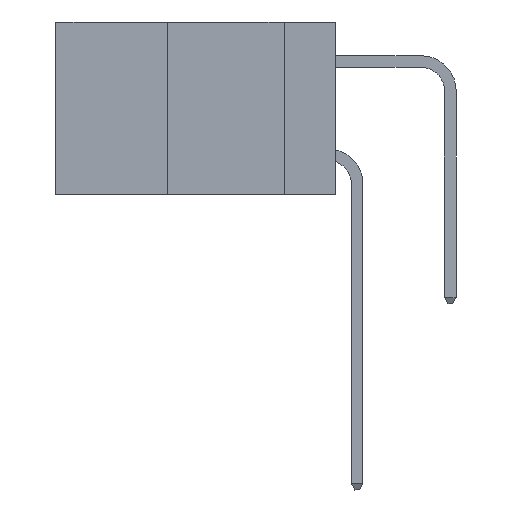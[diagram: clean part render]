
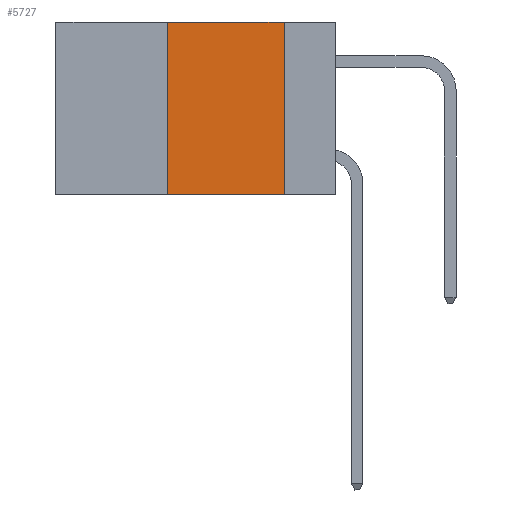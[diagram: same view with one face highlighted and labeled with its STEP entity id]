
A CAD part, left-side view. The second image highlights one B-rep face of the part: STEP entity #5727.
In plain terms, the highlighted planar face has unit normal (-1, 0, 0).
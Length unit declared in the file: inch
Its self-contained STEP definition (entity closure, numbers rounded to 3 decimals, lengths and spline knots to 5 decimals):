
#483 = VERTEX_POINT ( 'NONE', #3583 ) ;
#616 = DIRECTION ( 'NONE',  ( 1., 0., 0. ) ) ;
#626 = LINE ( 'NONE', #9694, #8537 ) ;
#1663 = ORIENTED_EDGE ( 'NONE', *, *, #20720, .F. ) ;
#2254 = LINE ( 'NONE', #4422, #19535 ) ;
#2584 = ORIENTED_EDGE ( 'NONE', *, *, #5345, .F. ) ;
#3583 = CARTESIAN_POINT ( 'NONE',  ( 0., 0.36, -0.37 ) ) ;
#4422 = CARTESIAN_POINT ( 'NONE',  ( 0., 0.11, 0. ) ) ;
#5345 = EDGE_CURVE ( 'NONE', #483, #9402, #626, .T. ) ;
#5434 = EDGE_CURVE ( 'NONE', #483, #13383, #18441, .T. ) ;
#5591 = FACE_OUTER_BOUND ( 'NONE', #19784, .T. ) ;
#5607 = CARTESIAN_POINT ( 'NONE',  ( 0., 0.6, 0. ) ) ;
#5727 = ADVANCED_FACE ( 'NONE', ( #5591 ), #17321, .F. ) ;
#5816 = ORIENTED_EDGE ( 'NONE', *, *, #11416, .F. ) ;
#7896 = CARTESIAN_POINT ( 'NONE',  ( 0., 0.11, 0. ) ) ;
#8312 = CARTESIAN_POINT ( 'NONE',  ( 0., 0.11, -0.37 ) ) ;
#8537 = VECTOR ( 'NONE', #13044, 39.37008 ) ;
#9402 = VERTEX_POINT ( 'NONE', #16211 ) ;
#9694 = CARTESIAN_POINT ( 'NONE',  ( 0., 0.36, 0. ) ) ;
#11203 = ORIENTED_EDGE ( 'NONE', *, *, #5434, .T. ) ;
#11416 = EDGE_CURVE ( 'NONE', #11446, #13383, #2254, .T. ) ;
#11446 = VERTEX_POINT ( 'NONE', #7896 ) ;
#12373 = DIRECTION ( 'NONE',  ( 0., 0., -1. ) ) ;
#13044 = DIRECTION ( 'NONE',  ( 0., 0., 1. ) ) ;
#13383 = VERTEX_POINT ( 'NONE', #8312 ) ;
#14866 = CARTESIAN_POINT ( 'NONE',  ( 0., 0.6, -0.37 ) ) ;
#15826 = VECTOR ( 'NONE', #21517, 39.37008 ) ;
#16211 = CARTESIAN_POINT ( 'NONE',  ( 0., 0.36, 0. ) ) ;
#17321 = PLANE ( 'NONE',  #19086 ) ;
#17823 = DIRECTION ( 'NONE',  ( 0., 0., -1. ) ) ;
#18287 = VECTOR ( 'NONE', #19466, 39.37008 ) ;
#18441 = LINE ( 'NONE', #14866, #15826 ) ;
#18801 = LINE ( 'NONE', #21039, #18287 ) ;
#19086 = AXIS2_PLACEMENT_3D ( 'NONE', #5607, #616, #12373 ) ;
#19466 = DIRECTION ( 'NONE',  ( 0., -1., 0. ) ) ;
#19535 = VECTOR ( 'NONE', #17823, 39.37008 ) ;
#19784 = EDGE_LOOP ( 'NONE', ( #5816, #1663, #2584, #11203 ) ) ;
#20720 = EDGE_CURVE ( 'NONE', #9402, #11446, #18801, .T. ) ;
#21039 = CARTESIAN_POINT ( 'NONE',  ( 0., 0.6, 0. ) ) ;
#21517 = DIRECTION ( 'NONE',  ( 0., -1., 0. ) ) ;
